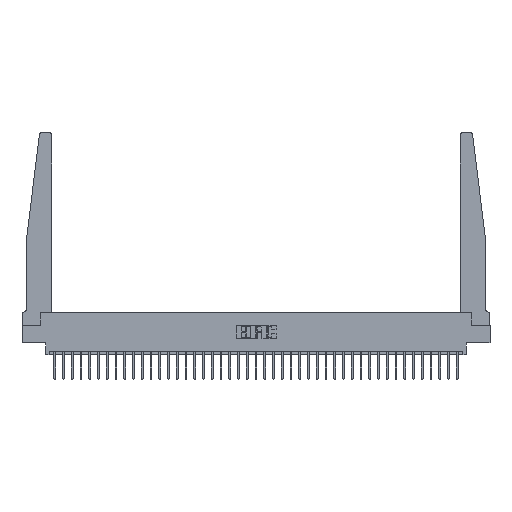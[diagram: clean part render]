
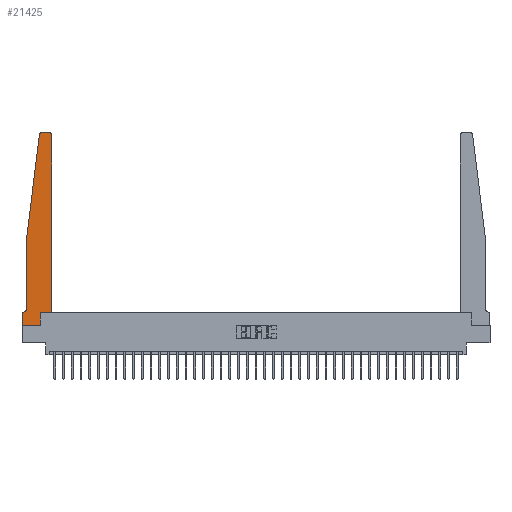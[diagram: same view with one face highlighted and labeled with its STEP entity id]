
A CAD part, top view. The second image highlights one B-rep face of the part: STEP entity #21425.
In plain terms, the highlighted planar face has unit normal (0, 0, 1).
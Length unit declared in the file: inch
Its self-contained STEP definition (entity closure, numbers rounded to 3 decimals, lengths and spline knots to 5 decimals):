
#113 = VECTOR ( 'NONE', #721, 39.37008 ) ;
#226 = CARTESIAN_POINT ( 'NONE',  ( 0.2605, 0., 0.37 ) ) ;
#697 = ORIENTED_EDGE ( 'NONE', *, *, #19891, .T. ) ;
#721 = DIRECTION ( 'NONE',  ( -0.122, -0.992, 0. ) ) ;
#1169 = DIRECTION ( 'NONE',  ( -1., 0., 0. ) ) ;
#1479 = VECTOR ( 'NONE', #23525, 39.37008 ) ;
#1817 = EDGE_CURVE ( 'NONE', #4387, #13551, #13883, .T. ) ;
#3030 = VERTEX_POINT ( 'NONE', #27667 ) ;
#3090 = CARTESIAN_POINT ( 'NONE',  ( 0.065, 1.25, 0.37 ) ) ;
#3166 = AXIS2_PLACEMENT_3D ( 'NONE', #29416, #13242, #32124 ) ;
#3263 = CARTESIAN_POINT ( 'NONE',  ( 0.015, 0.2375, 0.37 ) ) ;
#4081 = EDGE_CURVE ( 'NONE', #32509, #21076, #15839, .T. ) ;
#4132 = LINE ( 'NONE', #15301, #10457 ) ;
#4330 = VERTEX_POINT ( 'NONE', #22069 ) ;
#4387 = VERTEX_POINT ( 'NONE', #16743 ) ;
#4446 = CARTESIAN_POINT ( 'NONE',  ( 0.065, 0.1875, 0.37 ) ) ;
#4578 = DIRECTION ( 'NONE',  ( 1., 0., 0. ) ) ;
#4910 = LINE ( 'NONE', #16550, #11216 ) ;
#5213 = EDGE_CURVE ( 'NONE', #26931, #23400, #27600, .T. ) ;
#5832 = CARTESIAN_POINT ( 'NONE',  ( 0.015, 0.1875, 0.37 ) ) ;
#5971 = DIRECTION ( 'NONE',  ( -1., 0., 0. ) ) ;
#6187 = VECTOR ( 'NONE', #12587, 39.37008 ) ;
#6217 = CARTESIAN_POINT ( 'NONE',  ( 0., 0., 0.37 ) ) ;
#6449 = LINE ( 'NONE', #15427, #19961 ) ;
#7038 = DIRECTION ( 'NONE',  ( -1., 0., 0. ) ) ;
#7217 = CARTESIAN_POINT ( 'NONE',  ( 0.065, 0.2375, 0.37 ) ) ;
#7609 = ORIENTED_EDGE ( 'NONE', *, *, #28751, .T. ) ;
#7848 = VERTEX_POINT ( 'NONE', #3090 ) ;
#8143 = LINE ( 'NONE', #14134, #21659 ) ;
#8721 = VERTEX_POINT ( 'NONE', #6217 ) ;
#8772 = CARTESIAN_POINT ( 'NONE',  ( 0.065, 1.25, 0.37 ) ) ;
#9383 = AXIS2_PLACEMENT_3D ( 'NONE', #25675, #9500, #28384 ) ;
#9500 = DIRECTION ( 'NONE',  ( 0., 0., 1. ) ) ;
#9985 = ORIENTED_EDGE ( 'NONE', *, *, #16950, .T. ) ;
#10457 = VECTOR ( 'NONE', #4578, 39.37008 ) ;
#10843 = CIRCLE ( 'NONE', #13468, 0.05 ) ;
#11043 = FACE_OUTER_BOUND ( 'NONE', #29360, .T. ) ;
#11216 = VECTOR ( 'NONE', #21988, 39.37008 ) ;
#11829 = ORIENTED_EDGE ( 'NONE', *, *, #1817, .T. ) ;
#12587 = DIRECTION ( 'NONE',  ( 0., -1., 0. ) ) ;
#12807 = PLANE ( 'NONE',  #29408 ) ;
#13242 = DIRECTION ( 'NONE',  ( 0., 0., 1. ) ) ;
#13246 = ORIENTED_EDGE ( 'NONE', *, *, #29391, .T. ) ;
#13468 = AXIS2_PLACEMENT_3D ( 'NONE', #3263, #22146, #5971 ) ;
#13551 = VERTEX_POINT ( 'NONE', #22082 ) ;
#13883 = LINE ( 'NONE', #14612, #28279 ) ;
#14134 = CARTESIAN_POINT ( 'NONE',  ( 0.425, 0.18, 0.37 ) ) ;
#14612 = CARTESIAN_POINT ( 'NONE',  ( 0.25, 2.75, 0.37 ) ) ;
#15301 = CARTESIAN_POINT ( 'NONE',  ( 0., 0., 0.37 ) ) ;
#15427 = CARTESIAN_POINT ( 'NONE',  ( 0.065, 1.25, 0.37 ) ) ;
#15518 = DIRECTION ( 'NONE',  ( 0., 0., 1. ) ) ;
#15839 = LINE ( 'NONE', #20795, #1479 ) ;
#16550 = CARTESIAN_POINT ( 'NONE',  ( 0.425, 0.18, 0.37 ) ) ;
#16743 = CARTESIAN_POINT ( 'NONE',  ( 0.395, 2.75, 0.37 ) ) ;
#16838 = CARTESIAN_POINT ( 'NONE',  ( 0.2605, 0.18, 0.37 ) ) ;
#16950 = EDGE_CURVE ( 'NONE', #7848, #34275, #6449, .T. ) ;
#18666 = ORIENTED_EDGE ( 'NONE', *, *, #24660, .T. ) ;
#18873 = CARTESIAN_POINT ( 'NONE',  ( 0.425, 0.18, 0.37 ) ) ;
#19581 = DIRECTION ( 'NONE',  ( 1., 0., 0. ) ) ;
#19673 = EDGE_CURVE ( 'NONE', #13551, #3030, #27618, .T. ) ;
#19891 = EDGE_CURVE ( 'NONE', #3030, #7848, #28876, .T. ) ;
#19961 = VECTOR ( 'NONE', #34300, 39.37008 ) ;
#20368 = EDGE_CURVE ( 'NONE', #21076, #25458, #8143, .T. ) ;
#20520 = CIRCLE ( 'NONE', #9383, 0.03 ) ;
#20795 = CARTESIAN_POINT ( 'NONE',  ( 0.2605, 0.18, 0.37 ) ) ;
#21076 = VERTEX_POINT ( 'NONE', #16838 ) ;
#21425 = ADVANCED_FACE ( 'NONE', ( #11043 ), #12807, .T. ) ;
#21659 = VECTOR ( 'NONE', #19581, 39.37008 ) ;
#21879 = ORIENTED_EDGE ( 'NONE', *, *, #19673, .T. ) ;
#21988 = DIRECTION ( 'NONE',  ( 0., 1., 0. ) ) ;
#22069 = CARTESIAN_POINT ( 'NONE',  ( 0.425, 2.72, 0.37 ) ) ;
#22082 = CARTESIAN_POINT ( 'NONE',  ( 0.27653, 2.75, 0.37 ) ) ;
#22146 = DIRECTION ( 'NONE',  ( 0., 0., -1. ) ) ;
#23400 = VERTEX_POINT ( 'NONE', #32816 ) ;
#23525 = DIRECTION ( 'NONE',  ( 0., 1., 0. ) ) ;
#23836 = ORIENTED_EDGE ( 'NONE', *, *, #4081, .T. ) ;
#24660 = EDGE_CURVE ( 'NONE', #23400, #8721, #26873, .T. ) ;
#25106 = EDGE_CURVE ( 'NONE', #4330, #4387, #20520, .T. ) ;
#25458 = VERTEX_POINT ( 'NONE', #18873 ) ;
#25675 = CARTESIAN_POINT ( 'NONE',  ( 0.395, 2.72, 0.37 ) ) ;
#26688 = ORIENTED_EDGE ( 'NONE', *, *, #5213, .T. ) ;
#26873 = LINE ( 'NONE', #31460, #6187 ) ;
#26931 = VERTEX_POINT ( 'NONE', #5832 ) ;
#27600 = LINE ( 'NONE', #4446, #32208 ) ;
#27618 = CIRCLE ( 'NONE', #3166, 0.03 ) ;
#27667 = CARTESIAN_POINT ( 'NONE',  ( 0.24675, 2.72367, 0.37 ) ) ;
#28279 = VECTOR ( 'NONE', #1169, 39.37008 ) ;
#28384 = DIRECTION ( 'NONE',  ( 1., 0., 0. ) ) ;
#28497 = EDGE_CURVE ( 'NONE', #8721, #32509, #4132, .T. ) ;
#28751 = EDGE_CURVE ( 'NONE', #34275, #26931, #10843, .T. ) ;
#28876 = LINE ( 'NONE', #8772, #113 ) ;
#29360 = EDGE_LOOP ( 'NONE', ( #11829, #21879, #697, #9985, #7609, #26688, #18666, #32009, #23836, #32447, #13246, #33260 ) ) ;
#29391 = EDGE_CURVE ( 'NONE', #25458, #4330, #4910, .T. ) ;
#29408 = AXIS2_PLACEMENT_3D ( 'NONE', #31692, #15518, #34386 ) ;
#29416 = CARTESIAN_POINT ( 'NONE',  ( 0.27653, 2.72, 0.37 ) ) ;
#31460 = CARTESIAN_POINT ( 'NONE',  ( 0., 0., 0.37 ) ) ;
#31692 = CARTESIAN_POINT ( 'NONE',  ( 0., 0.1875, 0.37 ) ) ;
#32009 = ORIENTED_EDGE ( 'NONE', *, *, #28497, .T. ) ;
#32124 = DIRECTION ( 'NONE',  ( 1., 0., 0. ) ) ;
#32208 = VECTOR ( 'NONE', #7038, 39.37008 ) ;
#32447 = ORIENTED_EDGE ( 'NONE', *, *, #20368, .T. ) ;
#32509 = VERTEX_POINT ( 'NONE', #226 ) ;
#32816 = CARTESIAN_POINT ( 'NONE',  ( 0., 0.1875, 0.37 ) ) ;
#33260 = ORIENTED_EDGE ( 'NONE', *, *, #25106, .T. ) ;
#34275 = VERTEX_POINT ( 'NONE', #7217 ) ;
#34300 = DIRECTION ( 'NONE',  ( 0., -1., 0. ) ) ;
#34386 = DIRECTION ( 'NONE',  ( 1., 0., 0. ) ) ;
